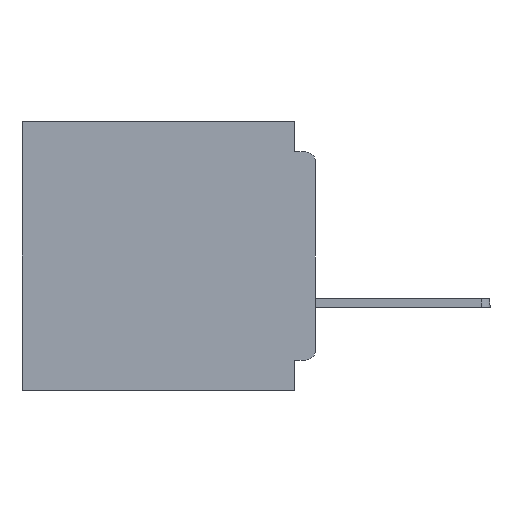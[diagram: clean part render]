
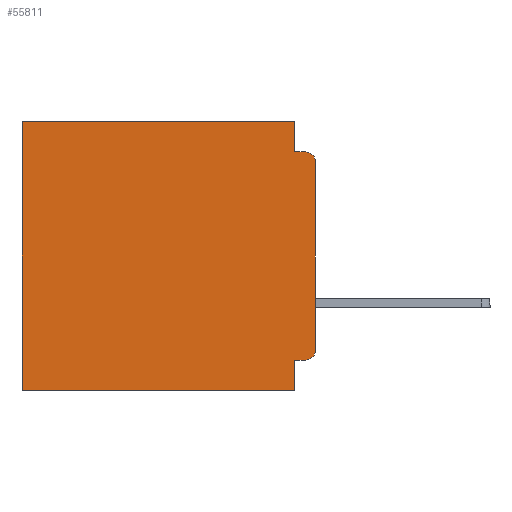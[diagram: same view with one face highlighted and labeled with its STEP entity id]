
A CAD part, left-side view. The second image highlights one B-rep face of the part: STEP entity #55811.
In plain terms, the highlighted planar face has unit normal (-1, 0, 0).
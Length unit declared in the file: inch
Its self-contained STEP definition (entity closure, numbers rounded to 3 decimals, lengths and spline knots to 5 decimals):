
#709 = DIRECTION ( 'NONE',  ( 0., 0., -1. ) ) ;
#1626 = EDGE_CURVE ( 'NONE', #27310, #14048, #57321, .T. ) ;
#1808 = AXIS2_PLACEMENT_3D ( 'NONE', #4992, #5536, #5446 ) ;
#4992 = CARTESIAN_POINT ( 'NONE',  ( 0.3, 0.015, -0.06 ) ) ;
#5380 = VECTOR ( 'NONE', #30501, 39.37008 ) ;
#5404 = CARTESIAN_POINT ( 'NONE',  ( 0.3, 0., -0.4 ) ) ;
#5446 = DIRECTION ( 'NONE',  ( 0., 0., -1. ) ) ;
#5455 = DIRECTION ( 'NONE',  ( 0., -1., 0. ) ) ;
#5536 = DIRECTION ( 'NONE',  ( -1., 0., 0. ) ) ;
#8128 = FACE_OUTER_BOUND ( 'NONE', #17520, .T. ) ;
#8890 = VERTEX_POINT ( 'NONE', #17576 ) ;
#11950 = ORIENTED_EDGE ( 'NONE', *, *, #13630, .T. ) ;
#12255 = EDGE_CURVE ( 'NONE', #54525, #50364, #18005, .T. ) ;
#12291 = CIRCLE ( 'NONE', #18768, 0.015 ) ;
#12606 = CARTESIAN_POINT ( 'NONE',  ( 0.3, 0.437, 0. ) ) ;
#13630 = EDGE_CURVE ( 'NONE', #54525, #17306, #19210, .T. ) ;
#14048 = VERTEX_POINT ( 'NONE', #45101 ) ;
#14113 = VERTEX_POINT ( 'NONE', #19863 ) ;
#15343 = VERTEX_POINT ( 'NONE', #65564 ) ;
#15735 = EDGE_CURVE ( 'NONE', #8890, #49516, #23787, .T. ) ;
#16674 = AXIS2_PLACEMENT_3D ( 'NONE', #61065, #66213, #35477 ) ;
#17051 = EDGE_CURVE ( 'NONE', #27310, #15343, #59768, .T. ) ;
#17306 = VERTEX_POINT ( 'NONE', #12606 ) ;
#17520 = EDGE_LOOP ( 'NONE', ( #24168, #66159, #35700, #66548, #11950, #56417, #62154, #48195, #21695, #19563 ) ) ;
#17576 = CARTESIAN_POINT ( 'NONE',  ( 0.3, 0.031, -0.355 ) ) ;
#18005 = LINE ( 'NONE', #52642, #43801 ) ;
#18698 = VECTOR ( 'NONE', #26021, 39.37008 ) ;
#18768 = AXIS2_PLACEMENT_3D ( 'NONE', #27752, #63712, #32948 ) ;
#19210 = LINE ( 'NONE', #66416, #5380 ) ;
#19563 = ORIENTED_EDGE ( 'NONE', *, *, #25187, .T. ) ;
#19863 = CARTESIAN_POINT ( 'NONE',  ( 0.3, 0.015, -0.355 ) ) ;
#20892 = CARTESIAN_POINT ( 'NONE',  ( 0.3, 0., -0.045 ) ) ;
#21415 = EDGE_CURVE ( 'NONE', #49516, #63140, #27425, .T. ) ;
#21695 = ORIENTED_EDGE ( 'NONE', *, *, #49099, .F. ) ;
#22430 = LINE ( 'NONE', #37014, #61843 ) ;
#23787 = LINE ( 'NONE', #38158, #49502 ) ;
#24168 = ORIENTED_EDGE ( 'NONE', *, *, #17051, .F. ) ;
#25131 = PLANE ( 'NONE',  #16674 ) ;
#25187 = EDGE_CURVE ( 'NONE', #14113, #15343, #12291, .T. ) ;
#25262 = CARTESIAN_POINT ( 'NONE',  ( 0.3, 0., -0.06 ) ) ;
#26021 = DIRECTION ( 'NONE',  ( 0., 0., -1. ) ) ;
#27310 = VERTEX_POINT ( 'NONE', #25262 ) ;
#27425 = LINE ( 'NONE', #5404, #42756 ) ;
#27752 = CARTESIAN_POINT ( 'NONE',  ( 0.3, 0.015, -0.34 ) ) ;
#30501 = DIRECTION ( 'NONE',  ( 0., 1., 0. ) ) ;
#32252 = VECTOR ( 'NONE', #5455, 39.37008 ) ;
#32318 = VECTOR ( 'NONE', #40616, 39.37008 ) ;
#32948 = DIRECTION ( 'NONE',  ( 0., 0., -1. ) ) ;
#35005 = CARTESIAN_POINT ( 'NONE',  ( 0.3, 0.031, -0.045 ) ) ;
#35477 = DIRECTION ( 'NONE',  ( 0., 0., -1. ) ) ;
#35700 = ORIENTED_EDGE ( 'NONE', *, *, #57099, .F. ) ;
#37014 = CARTESIAN_POINT ( 'NONE',  ( 0.3, 0.437, -0.4 ) ) ;
#38158 = CARTESIAN_POINT ( 'NONE',  ( 0.3, 0.031, -0.4 ) ) ;
#38766 = CARTESIAN_POINT ( 'NONE',  ( 0.3, 0.031, 0. ) ) ;
#40616 = DIRECTION ( 'NONE',  ( 0., 1., 0. ) ) ;
#42756 = VECTOR ( 'NONE', #46490, 39.37008 ) ;
#43331 = DIRECTION ( 'NONE',  ( 0., 0., -1. ) ) ;
#43801 = VECTOR ( 'NONE', #57845, 39.37008 ) ;
#45101 = CARTESIAN_POINT ( 'NONE',  ( 0.3, 0.015, -0.045 ) ) ;
#45928 = LINE ( 'NONE', #20892, #32252 ) ;
#46465 = CARTESIAN_POINT ( 'NONE',  ( 0.3, 0., -0.4 ) ) ;
#46490 = DIRECTION ( 'NONE',  ( 0., 1., 0. ) ) ;
#48195 = ORIENTED_EDGE ( 'NONE', *, *, #15735, .F. ) ;
#49058 = CARTESIAN_POINT ( 'NONE',  ( 0.3, 0.031, -0.4 ) ) ;
#49099 = EDGE_CURVE ( 'NONE', #14113, #8890, #59669, .T. ) ;
#49502 = VECTOR ( 'NONE', #43331, 39.37008 ) ;
#49516 = VERTEX_POINT ( 'NONE', #49058 ) ;
#50364 = VERTEX_POINT ( 'NONE', #35005 ) ;
#50625 = EDGE_CURVE ( 'NONE', #17306, #63140, #22430, .T. ) ;
#52642 = CARTESIAN_POINT ( 'NONE',  ( 0.3, 0.031, 0. ) ) ;
#54525 = VERTEX_POINT ( 'NONE', #38766 ) ;
#55811 = ADVANCED_FACE ( 'NONE', ( #8128 ), #25131, .F. ) ;
#56417 = ORIENTED_EDGE ( 'NONE', *, *, #50625, .T. ) ;
#57099 = EDGE_CURVE ( 'NONE', #50364, #14048, #45928, .T. ) ;
#57321 = CIRCLE ( 'NONE', #1808, 0.015 ) ;
#57845 = DIRECTION ( 'NONE',  ( 0., 0., -1. ) ) ;
#59669 = LINE ( 'NONE', #66133, #32318 ) ;
#59768 = LINE ( 'NONE', #46465, #18698 ) ;
#61065 = CARTESIAN_POINT ( 'NONE',  ( 0.3, 0., -0.4 ) ) ;
#61843 = VECTOR ( 'NONE', #709, 39.37008 ) ;
#62154 = ORIENTED_EDGE ( 'NONE', *, *, #21415, .F. ) ;
#63140 = VERTEX_POINT ( 'NONE', #63961 ) ;
#63712 = DIRECTION ( 'NONE',  ( -1., 0., 0. ) ) ;
#63961 = CARTESIAN_POINT ( 'NONE',  ( 0.3, 0.437, -0.4 ) ) ;
#65564 = CARTESIAN_POINT ( 'NONE',  ( 0.3, 0., -0.34 ) ) ;
#66133 = CARTESIAN_POINT ( 'NONE',  ( 0.3, 0., -0.355 ) ) ;
#66159 = ORIENTED_EDGE ( 'NONE', *, *, #1626, .T. ) ;
#66213 = DIRECTION ( 'NONE',  ( 1., 0., 0. ) ) ;
#66416 = CARTESIAN_POINT ( 'NONE',  ( 0.3, 0., 0. ) ) ;
#66548 = ORIENTED_EDGE ( 'NONE', *, *, #12255, .F. ) ;
